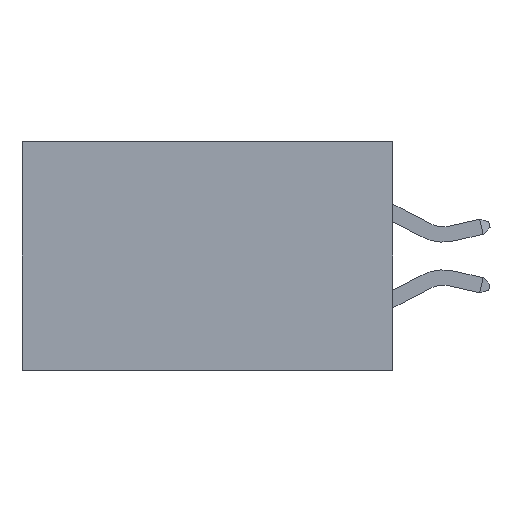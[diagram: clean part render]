
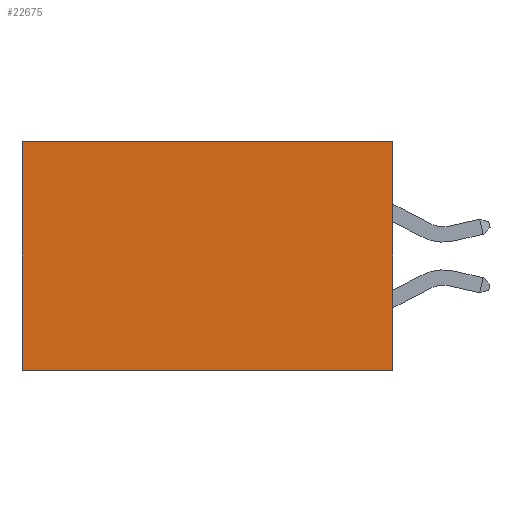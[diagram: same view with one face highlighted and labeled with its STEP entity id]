
A CAD part, left-side view. The second image highlights one B-rep face of the part: STEP entity #22675.
In plain terms, the highlighted planar face has unit normal (-1, 0, 0).
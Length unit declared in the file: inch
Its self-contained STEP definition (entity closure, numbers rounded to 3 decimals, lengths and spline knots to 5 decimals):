
#286 = CARTESIAN_POINT ( 'NONE',  ( 0.2875, 0., 0. ) ) ;
#1535 = ORIENTED_EDGE ( 'NONE', *, *, #8709, .T. ) ;
#1856 = LINE ( 'NONE', #5433, #26859 ) ;
#2403 = EDGE_CURVE ( 'NONE', #19604, #23588, #4989, .T. ) ;
#3281 = DIRECTION ( 'NONE',  ( 0., 0., -1. ) ) ;
#3733 = VERTEX_POINT ( 'NONE', #13705 ) ;
#4239 = CARTESIAN_POINT ( 'NONE',  ( 0.2875, 0., -0.37 ) ) ;
#4989 = LINE ( 'NONE', #20084, #7313 ) ;
#5433 = CARTESIAN_POINT ( 'NONE',  ( 0.2875, 0.6, 0. ) ) ;
#6646 = AXIS2_PLACEMENT_3D ( 'NONE', #24791, #16359, #12123 ) ;
#7288 = VECTOR ( 'NONE', #21984, 39.37008 ) ;
#7313 = VECTOR ( 'NONE', #3281, 39.37008 ) ;
#8083 = VECTOR ( 'NONE', #23113, 39.37008 ) ;
#8709 = EDGE_CURVE ( 'NONE', #19604, #25473, #12875, .T. ) ;
#9939 = EDGE_LOOP ( 'NONE', ( #18741, #22954, #21417, #1535 ) ) ;
#10712 = CARTESIAN_POINT ( 'NONE',  ( 0.2875, 0., -0.37 ) ) ;
#10741 = FACE_OUTER_BOUND ( 'NONE', #9939, .T. ) ;
#11259 = EDGE_CURVE ( 'NONE', #25473, #3733, #1856, .T. ) ;
#12123 = DIRECTION ( 'NONE',  ( 0., 0., -1. ) ) ;
#12875 = LINE ( 'NONE', #19248, #7288 ) ;
#13484 = EDGE_CURVE ( 'NONE', #23588, #3733, #13602, .T. ) ;
#13602 = LINE ( 'NONE', #10712, #8083 ) ;
#13705 = CARTESIAN_POINT ( 'NONE',  ( 0.2875, 0.6, -0.37 ) ) ;
#16359 = DIRECTION ( 'NONE',  ( 1., 0., 0. ) ) ;
#17201 = CARTESIAN_POINT ( 'NONE',  ( 0.2875, 0.6, 0. ) ) ;
#18741 = ORIENTED_EDGE ( 'NONE', *, *, #11259, .T. ) ;
#19248 = CARTESIAN_POINT ( 'NONE',  ( 0.2875, 0., 0. ) ) ;
#19604 = VERTEX_POINT ( 'NONE', #286 ) ;
#20084 = CARTESIAN_POINT ( 'NONE',  ( 0.2875, 0., 0. ) ) ;
#20671 = PLANE ( 'NONE',  #6646 ) ;
#21417 = ORIENTED_EDGE ( 'NONE', *, *, #2403, .F. ) ;
#21984 = DIRECTION ( 'NONE',  ( 0., 1., 0. ) ) ;
#22543 = DIRECTION ( 'NONE',  ( 0., 0., -1. ) ) ;
#22675 = ADVANCED_FACE ( 'NONE', ( #10741 ), #20671, .F. ) ;
#22954 = ORIENTED_EDGE ( 'NONE', *, *, #13484, .F. ) ;
#23113 = DIRECTION ( 'NONE',  ( 0., 1., 0. ) ) ;
#23588 = VERTEX_POINT ( 'NONE', #4239 ) ;
#24791 = CARTESIAN_POINT ( 'NONE',  ( 0.2875, 0., 0. ) ) ;
#25473 = VERTEX_POINT ( 'NONE', #17201 ) ;
#26859 = VECTOR ( 'NONE', #22543, 39.37008 ) ;
